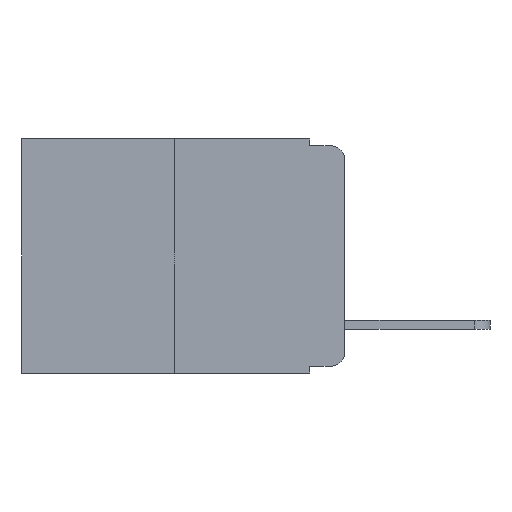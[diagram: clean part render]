
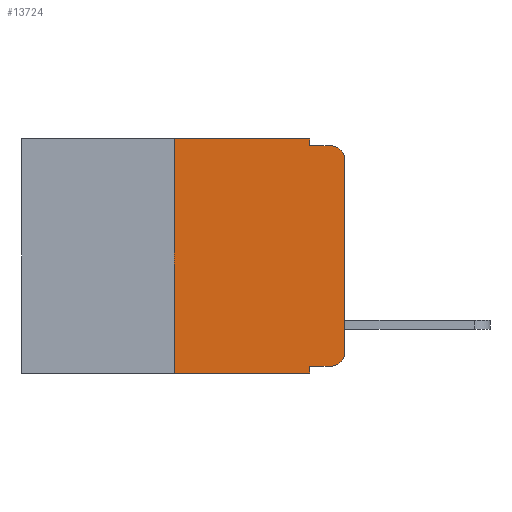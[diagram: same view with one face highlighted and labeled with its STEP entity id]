
A CAD part, left-side view. The second image highlights one B-rep face of the part: STEP entity #13724.
In plain terms, the highlighted planar face has unit normal (-1, 0, 0).
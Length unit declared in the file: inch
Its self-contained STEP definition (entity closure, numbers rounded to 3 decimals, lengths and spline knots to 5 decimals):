
#27 = VERTEX_POINT ( 'NONE', #7729 ) ;
#95 = VECTOR ( 'NONE', #13481, 39.37008 ) ;
#202 = EDGE_CURVE ( 'NONE', #17502, #17704, #17421, .T. ) ;
#307 = CARTESIAN_POINT ( 'NONE',  ( 0., 0.473, -0.343 ) ) ;
#423 = CARTESIAN_POINT ( 'NONE',  ( 0., 0.051, -0.333 ) ) ;
#523 = PLANE ( 'NONE',  #10366 ) ;
#693 = EDGE_CURVE ( 'NONE', #4223, #27, #814, .T. ) ;
#814 = CIRCLE ( 'NONE', #9855, 0.02 ) ;
#1863 = DIRECTION ( 'NONE',  ( 1., 0., 0. ) ) ;
#2006 = AXIS2_PLACEMENT_3D ( 'NONE', #4282, #5671, #15884 ) ;
#2293 = EDGE_CURVE ( 'NONE', #9523, #17171, #18471, .T. ) ;
#2332 = LINE ( 'NONE', #4056, #17303 ) ;
#2379 = VECTOR ( 'NONE', #13636, 39.37008 ) ;
#2526 = VECTOR ( 'NONE', #5020, 39.37008 ) ;
#3092 = VERTEX_POINT ( 'NONE', #423 ) ;
#3319 = ORIENTED_EDGE ( 'NONE', *, *, #16778, .T. ) ;
#3347 = DIRECTION ( 'NONE',  ( 0., 0., -1. ) ) ;
#4056 = CARTESIAN_POINT ( 'NONE',  ( 0., 0.25, 0. ) ) ;
#4223 = VERTEX_POINT ( 'NONE', #18735 ) ;
#4282 = CARTESIAN_POINT ( 'NONE',  ( 0., 0.02, -0.03 ) ) ;
#4343 = CARTESIAN_POINT ( 'NONE',  ( 0., 0., -0.03 ) ) ;
#4439 = CARTESIAN_POINT ( 'NONE',  ( 0., 0.051, -0.343 ) ) ;
#4619 = VERTEX_POINT ( 'NONE', #17077 ) ;
#5020 = DIRECTION ( 'NONE',  ( 0., -1., 0. ) ) ;
#5506 = CARTESIAN_POINT ( 'NONE',  ( 0., 0.051, 0. ) ) ;
#5671 = DIRECTION ( 'NONE',  ( -1., 0., 0. ) ) ;
#6224 = LINE ( 'NONE', #15197, #2379 ) ;
#6393 = ORIENTED_EDGE ( 'NONE', *, *, #2293, .F. ) ;
#6717 = ORIENTED_EDGE ( 'NONE', *, *, #202, .F. ) ;
#7046 = EDGE_CURVE ( 'NONE', #3092, #4223, #8426, .T. ) ;
#7094 = CARTESIAN_POINT ( 'NONE',  ( 0., 0.02, -0.313 ) ) ;
#7729 = CARTESIAN_POINT ( 'NONE',  ( 0., 0., -0.313 ) ) ;
#8426 = LINE ( 'NONE', #12271, #2526 ) ;
#8568 = DIRECTION ( 'NONE',  ( -1., 0., 0. ) ) ;
#8694 = VECTOR ( 'NONE', #11932, 39.37008 ) ;
#8754 = VECTOR ( 'NONE', #3347, 39.37008 ) ;
#8861 = EDGE_LOOP ( 'NONE', ( #13972, #16098, #6717, #15060, #6393, #14210, #3319, #16908, #12461, #15665 ) ) ;
#8924 = CARTESIAN_POINT ( 'NONE',  ( 0., 0.051, 0. ) ) ;
#9182 = CIRCLE ( 'NONE', #2006, 0.02 ) ;
#9523 = VERTEX_POINT ( 'NONE', #13609 ) ;
#9855 = AXIS2_PLACEMENT_3D ( 'NONE', #7094, #8568, #18711 ) ;
#9945 = DIRECTION ( 'NONE',  ( 0., -1., 0. ) ) ;
#10366 = AXIS2_PLACEMENT_3D ( 'NONE', #16390, #1863, #13618 ) ;
#10753 = EDGE_CURVE ( 'NONE', #27, #13581, #17394, .T. ) ;
#11077 = EDGE_CURVE ( 'NONE', #13581, #17704, #9182, .T. ) ;
#11268 = CARTESIAN_POINT ( 'NONE',  ( 0., 0.051, -0.01 ) ) ;
#11932 = DIRECTION ( 'NONE',  ( 0., -1., 0. ) ) ;
#12271 = CARTESIAN_POINT ( 'NONE',  ( 0., 0.051, -0.333 ) ) ;
#12461 = ORIENTED_EDGE ( 'NONE', *, *, #7046, .T. ) ;
#12613 = LINE ( 'NONE', #8924, #8754 ) ;
#12643 = VECTOR ( 'NONE', #15508, 39.37008 ) ;
#12690 = DIRECTION ( 'NONE',  ( 0., 0., 1. ) ) ;
#13481 = DIRECTION ( 'NONE',  ( 0., 0., 1. ) ) ;
#13581 = VERTEX_POINT ( 'NONE', #4343 ) ;
#13609 = CARTESIAN_POINT ( 'NONE',  ( 0., 0.25, 0. ) ) ;
#13618 = DIRECTION ( 'NONE',  ( 0., 0., -1. ) ) ;
#13636 = DIRECTION ( 'NONE',  ( 0., 0., -1. ) ) ;
#13724 = ADVANCED_FACE ( 'NONE', ( #15388 ), #523, .F. ) ;
#13972 = ORIENTED_EDGE ( 'NONE', *, *, #10753, .T. ) ;
#14210 = ORIENTED_EDGE ( 'NONE', *, *, #17154, .F. ) ;
#14587 = VECTOR ( 'NONE', #9945, 39.37008 ) ;
#14695 = VERTEX_POINT ( 'NONE', #4439 ) ;
#14863 = CARTESIAN_POINT ( 'NONE',  ( 0., 0., 0. ) ) ;
#15060 = ORIENTED_EDGE ( 'NONE', *, *, #15653, .F. ) ;
#15197 = CARTESIAN_POINT ( 'NONE',  ( 0., 0.051, 0. ) ) ;
#15388 = FACE_OUTER_BOUND ( 'NONE', #8861, .T. ) ;
#15486 = LINE ( 'NONE', #307, #8694 ) ;
#15508 = DIRECTION ( 'NONE',  ( 0., -1., 0. ) ) ;
#15529 = EDGE_CURVE ( 'NONE', #3092, #14695, #12613, .T. ) ;
#15653 = EDGE_CURVE ( 'NONE', #17171, #17502, #6224, .T. ) ;
#15665 = ORIENTED_EDGE ( 'NONE', *, *, #693, .T. ) ;
#15870 = CARTESIAN_POINT ( 'NONE',  ( 0., 0.02, -0.01 ) ) ;
#15884 = DIRECTION ( 'NONE',  ( 0., 0., -1. ) ) ;
#16098 = ORIENTED_EDGE ( 'NONE', *, *, #11077, .T. ) ;
#16390 = CARTESIAN_POINT ( 'NONE',  ( 0., 0.473, 0. ) ) ;
#16778 = EDGE_CURVE ( 'NONE', #4619, #14695, #15486, .T. ) ;
#16908 = ORIENTED_EDGE ( 'NONE', *, *, #15529, .F. ) ;
#17077 = CARTESIAN_POINT ( 'NONE',  ( 0., 0.25, -0.343 ) ) ;
#17154 = EDGE_CURVE ( 'NONE', #4619, #9523, #2332, .T. ) ;
#17171 = VERTEX_POINT ( 'NONE', #5506 ) ;
#17194 = CARTESIAN_POINT ( 'NONE',  ( 0., 0.473, 0. ) ) ;
#17303 = VECTOR ( 'NONE', #12690, 39.37008 ) ;
#17394 = LINE ( 'NONE', #14863, #95 ) ;
#17421 = LINE ( 'NONE', #11268, #12643 ) ;
#17502 = VERTEX_POINT ( 'NONE', #18146 ) ;
#17704 = VERTEX_POINT ( 'NONE', #15870 ) ;
#18146 = CARTESIAN_POINT ( 'NONE',  ( 0., 0.051, -0.01 ) ) ;
#18471 = LINE ( 'NONE', #17194, #14587 ) ;
#18711 = DIRECTION ( 'NONE',  ( 0., 0., -1. ) ) ;
#18735 = CARTESIAN_POINT ( 'NONE',  ( 0., 0.02, -0.333 ) ) ;
